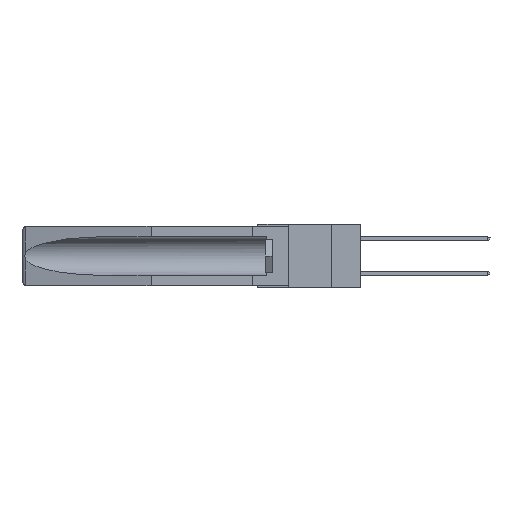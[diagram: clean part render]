
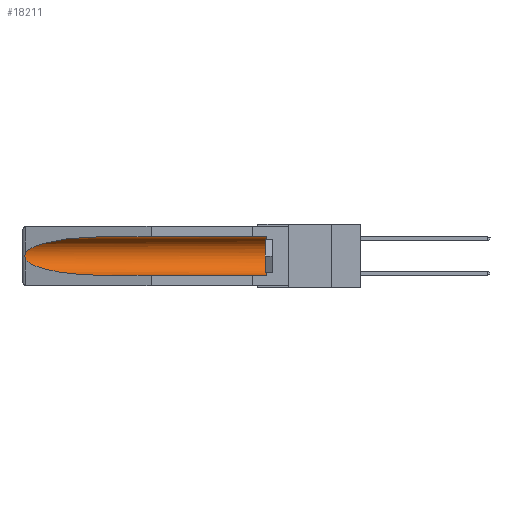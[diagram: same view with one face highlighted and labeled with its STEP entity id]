
A CAD part, left-side view. The second image highlights one B-rep face of the part: STEP entity #18211.
In plain terms, the highlighted cylindrical face has radius 2.857 mm (diameter 5.715 mm), a partial arc.
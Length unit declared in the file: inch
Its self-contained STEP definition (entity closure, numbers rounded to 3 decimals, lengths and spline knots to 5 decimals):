
#36 = CARTESIAN_POINT ( 'NONE',  ( 0.26537, 1.52718, -0.14972 ) ) ;
#410 = CARTESIAN_POINT ( 'NONE',  ( 0.2675, 1.53308, -0.17534 ) ) ;
#1505 = VECTOR ( 'NONE', #5870, 39.37008 ) ;
#1953 = CARTESIAN_POINT ( 'NONE',  ( 0.155, 1.07973, -0.059 ) ) ;
#2123 = VERTEX_POINT ( 'NONE', #9499 ) ;
#2367 = CARTESIAN_POINT ( 'NONE',  ( 0.155, -0.30754, -0.1715 ) ) ;
#2463 =( BOUNDED_CURVE ( )  B_SPLINE_CURVE ( 3, ( #1953, #8202, #8297, #36 ),
 .UNSPECIFIED., .F., .F. ) 
 B_SPLINE_CURVE_WITH_KNOTS ( ( 4, 4 ),
 ( 4.71239, 6.08839 ),
 .UNSPECIFIED. ) 
 CURVE ( )  GEOMETRIC_REPRESENTATION_ITEM ( )  RATIONAL_B_SPLINE_CURVE ( ( 1., 0.848, 0.848, 1. ) ) 
 REPRESENTATION_ITEM ( '' )  );
#2482 = CARTESIAN_POINT ( 'NONE',  ( 0.26537, 1.52718, -0.19328 ) ) ;
#2565 = CARTESIAN_POINT ( 'NONE',  ( 0.155, -0.30754, -0.284 ) ) ;
#2584 = CARTESIAN_POINT ( 'NONE',  ( 0.26597, 1.5296, -0.19026 ) ) ;
#3154 = ORIENTED_EDGE ( 'NONE', *, *, #10727, .T. ) ;
#4263 = CARTESIAN_POINT ( 'NONE',  ( 0.2675, 1.53308, -0.16763 ) ) ;
#5869 = CARTESIAN_POINT ( 'NONE',  ( 0.155, 0.126, -0.284 ) ) ;
#5870 = DIRECTION ( 'NONE',  ( 0., 1., 0. ) ) ;
#6500 = CARTESIAN_POINT ( 'NONE',  ( 0.25451, 1.48313, -0.24835 ) ) ;
#6566 = AXIS2_PLACEMENT_3D ( 'NONE', #2367, #24725, #20721 ) ;
#7159 = VERTEX_POINT ( 'NONE', #12985 ) ;
#7830 = CARTESIAN_POINT ( 'NONE',  ( 0.155, 0.126, -0.1715 ) ) ;
#8202 = CARTESIAN_POINT ( 'NONE',  ( 0.21114, 1.30732, -0.059 ) ) ;
#8297 = CARTESIAN_POINT ( 'NONE',  ( 0.25451, 1.48313, -0.09465 ) ) ;
#8307 = ORIENTED_EDGE ( 'NONE', *, *, #22089, .F. ) ;
#8672 = CARTESIAN_POINT ( 'NONE',  ( 0.26655, 1.53094, -0.18657 ) ) ;
#8694 = AXIS2_PLACEMENT_3D ( 'NONE', #7830, #19852, #15961 ) ;
#9499 = CARTESIAN_POINT ( 'NONE',  ( 0.26537, 1.52718, -0.14972 ) ) ;
#9981 = VECTOR ( 'NONE', #18714, 39.37008 ) ;
#10028 = CARTESIAN_POINT ( 'NONE',  ( 0.155, 1.07973, -0.284 ) ) ;
#10402 = EDGE_CURVE ( 'NONE', #24891, #21373, #10688, .T. ) ;
#10468 = CARTESIAN_POINT ( 'NONE',  ( 0.26654, 1.53092, -0.15636 ) ) ;
#10688 = CIRCLE ( 'NONE', #8694, 0.1125 ) ;
#10727 = EDGE_CURVE ( 'NONE', #21373, #7159, #19822, .T. ) ;
#12648 = CARTESIAN_POINT ( 'NONE',  ( 0.155, 1.07973, -0.284 ) ) ;
#12985 = CARTESIAN_POINT ( 'NONE',  ( 0.155, 1.07973, -0.059 ) ) ;
#13204 = CARTESIAN_POINT ( 'NONE',  ( 0.155, 0.126, -0.059 ) ) ;
#13391 = EDGE_CURVE ( 'NONE', #2123, #24889, #20904, .T. ) ;
#13924 = CYLINDRICAL_SURFACE ( 'NONE', #6566, 0.1125 ) ;
#14092 = EDGE_CURVE ( 'NONE', #7159, #2123, #2463, .T. ) ;
#14686 = CARTESIAN_POINT ( 'NONE',  ( 0.26537, 1.52718, -0.14972 ) ) ;
#15961 = DIRECTION ( 'NONE',  ( 0., 0., 1. ) ) ;
#17822 = EDGE_CURVE ( 'NONE', #24889, #21870, #21235, .T. ) ;
#18211 = ADVANCED_FACE ( 'NONE', ( #25316 ), #13924, .F. ) ;
#18478 = CARTESIAN_POINT ( 'NONE',  ( 0.26597, 1.52961, -0.15275 ) ) ;
#18540 = ORIENTED_EDGE ( 'NONE', *, *, #17822, .T. ) ;
#18714 = DIRECTION ( 'NONE',  ( 0., 1., 0. ) ) ;
#19822 = LINE ( 'NONE', #19943, #1505 ) ;
#19852 = DIRECTION ( 'NONE',  ( 0., -1., 0. ) ) ;
#19943 = CARTESIAN_POINT ( 'NONE',  ( 0.155, -0.30754, -0.059 ) ) ;
#20384 = EDGE_LOOP ( 'NONE', ( #22479, #21436, #18540, #8307, #24912, #3154 ) ) ;
#20604 = CARTESIAN_POINT ( 'NONE',  ( 0.26537, 1.52718, -0.19328 ) ) ;
#20667 = CARTESIAN_POINT ( 'NONE',  ( 0.21114, 1.30732, -0.284 ) ) ;
#20721 = DIRECTION ( 'NONE',  ( 0., 0., 1. ) ) ;
#20904 = B_SPLINE_CURVE_WITH_KNOTS ( 'NONE', 3,
 ( #14686, #18478, #10468, #24612, #4263, #410, #24697, #8672, #2584, #20604 ),
 .UNSPECIFIED., .F., .F.,
 ( 4, 2, 2, 2, 4 ),
 ( 0., 0.00029, 0.00058, 0.00087, 0.00117 ),
 .UNSPECIFIED. ) ;
#21235 =( BOUNDED_CURVE ( )  B_SPLINE_CURVE ( 3, ( #2482, #6500, #20667, #12648 ),
 .UNSPECIFIED., .F., .F. ) 
 B_SPLINE_CURVE_WITH_KNOTS ( ( 4, 4 ),
 ( 0.1948, 1.5708 ),
 .UNSPECIFIED. ) 
 CURVE ( )  GEOMETRIC_REPRESENTATION_ITEM ( )  RATIONAL_B_SPLINE_CURVE ( ( 1., 0.848, 0.848, 1. ) ) 
 REPRESENTATION_ITEM ( '' )  );
#21362 = LINE ( 'NONE', #2565, #9981 ) ;
#21373 = VERTEX_POINT ( 'NONE', #13204 ) ;
#21436 = ORIENTED_EDGE ( 'NONE', *, *, #13391, .T. ) ;
#21870 = VERTEX_POINT ( 'NONE', #10028 ) ;
#22089 = EDGE_CURVE ( 'NONE', #24891, #21870, #21362, .T. ) ;
#22479 = ORIENTED_EDGE ( 'NONE', *, *, #14092, .T. ) ;
#24612 = CARTESIAN_POINT ( 'NONE',  ( 0.2673, 1.5327, -0.16383 ) ) ;
#24697 = CARTESIAN_POINT ( 'NONE',  ( 0.2673, 1.53269, -0.17917 ) ) ;
#24725 = DIRECTION ( 'NONE',  ( 0., 1., 0. ) ) ;
#24889 = VERTEX_POINT ( 'NONE', #25780 ) ;
#24891 = VERTEX_POINT ( 'NONE', #5869 ) ;
#24912 = ORIENTED_EDGE ( 'NONE', *, *, #10402, .T. ) ;
#25316 = FACE_OUTER_BOUND ( 'NONE', #20384, .T. ) ;
#25780 = CARTESIAN_POINT ( 'NONE',  ( 0.26537, 1.52718, -0.19328 ) ) ;
